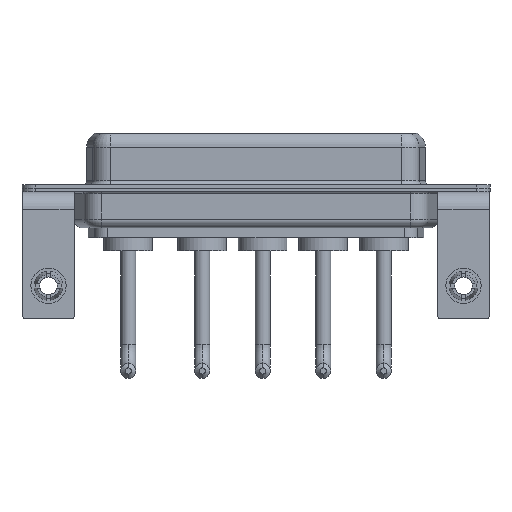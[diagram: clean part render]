
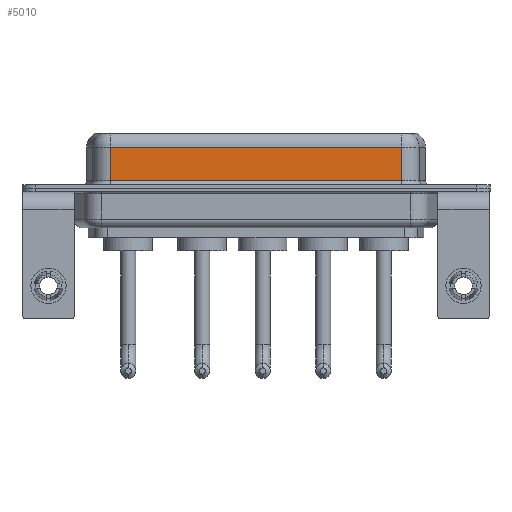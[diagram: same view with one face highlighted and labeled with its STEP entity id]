
A CAD part, front view. The second image highlights one B-rep face of the part: STEP entity #5010.
In plain terms, the highlighted planar face has unit normal (0, -1, 0).
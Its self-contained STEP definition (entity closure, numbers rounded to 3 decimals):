
#175 = CARTESIAN_POINT ( 'NONE',  ( 7.013, -3.95, 4.65 ) ) ;
#246 = VERTEX_POINT ( 'NONE', #8351 ) ;
#667 = CARTESIAN_POINT ( 'NONE',  ( 40.037, -3.95, 6.4 ) ) ;
#892 = DIRECTION ( 'NONE',  ( 0., 0., -1. ) ) ;
#1027 = EDGE_CURVE ( 'NONE', #246, #13763, #12672, .T. ) ;
#1814 = CARTESIAN_POINT ( 'NONE',  ( 7.013, -3.95, 0.9 ) ) ;
#1845 = ORIENTED_EDGE ( 'NONE', *, *, #12755, .T. ) ;
#3345 = VERTEX_POINT ( 'NONE', #1814 ) ;
#3389 = LINE ( 'NONE', #11611, #9469 ) ;
#3524 = ORIENTED_EDGE ( 'NONE', *, *, #1027, .T. ) ;
#3881 = CARTESIAN_POINT ( 'NONE',  ( 40.037, -3.95, 0.9 ) ) ;
#4568 = CARTESIAN_POINT ( 'NONE',  ( 40.037, -3.95, 6.4 ) ) ;
#5010 = ADVANCED_FACE ( 'NONE', ( #13892 ), #10572, .F. ) ;
#5675 = DIRECTION ( 'NONE',  ( 1., 0., 0. ) ) ;
#6366 = EDGE_CURVE ( 'NONE', #3345, #12417, #3389, .T. ) ;
#7110 = ORIENTED_EDGE ( 'NONE', *, *, #12492, .F. ) ;
#7299 = LINE ( 'NONE', #11940, #12328 ) ;
#7926 = CARTESIAN_POINT ( 'NONE',  ( 40.037, -3.95, 4.65 ) ) ;
#8237 = ORIENTED_EDGE ( 'NONE', *, *, #6366, .T. ) ;
#8351 = CARTESIAN_POINT ( 'NONE',  ( 40.037, -3.95, 4.65 ) ) ;
#8567 = VECTOR ( 'NONE', #13579, 1000. ) ;
#9133 = EDGE_LOOP ( 'NONE', ( #7110, #3524, #1845, #8237 ) ) ;
#9469 = VECTOR ( 'NONE', #5675, 1000. ) ;
#10109 = LINE ( 'NONE', #667, #14775 ) ;
#10499 = DIRECTION ( 'NONE',  ( 0., 0., 1. ) ) ;
#10572 = PLANE ( 'NONE',  #14081 ) ;
#11611 = CARTESIAN_POINT ( 'NONE',  ( 40.037, -3.95, 0.9 ) ) ;
#11940 = CARTESIAN_POINT ( 'NONE',  ( 7.013, -3.95, 6.4 ) ) ;
#12086 = DIRECTION ( 'NONE',  ( 0., 0., -1. ) ) ;
#12328 = VECTOR ( 'NONE', #12086, 1000. ) ;
#12417 = VERTEX_POINT ( 'NONE', #3881 ) ;
#12492 = EDGE_CURVE ( 'NONE', #246, #12417, #10109, .T. ) ;
#12672 = LINE ( 'NONE', #7926, #8567 ) ;
#12755 = EDGE_CURVE ( 'NONE', #13763, #3345, #7299, .T. ) ;
#12817 = DIRECTION ( 'NONE',  ( 0., 1., 0. ) ) ;
#13579 = DIRECTION ( 'NONE',  ( -1., 0., 0. ) ) ;
#13763 = VERTEX_POINT ( 'NONE', #175 ) ;
#13892 = FACE_OUTER_BOUND ( 'NONE', #9133, .T. ) ;
#14081 = AXIS2_PLACEMENT_3D ( 'NONE', #4568, #12817, #10499 ) ;
#14775 = VECTOR ( 'NONE', #892, 1000. ) ;
